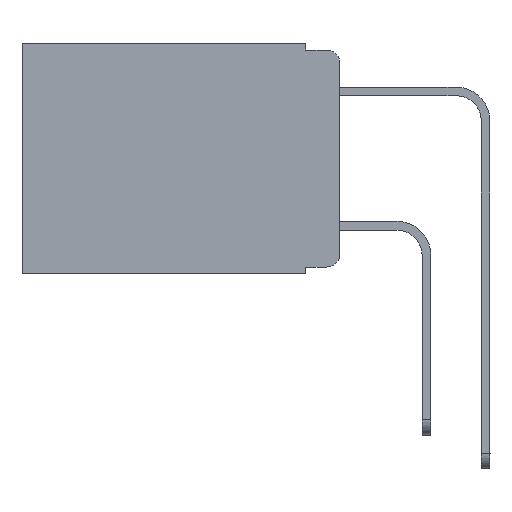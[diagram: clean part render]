
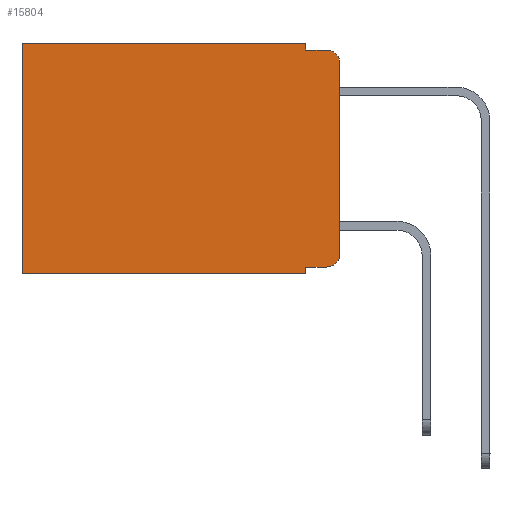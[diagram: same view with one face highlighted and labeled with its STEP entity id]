
A CAD part, left-side view. The second image highlights one B-rep face of the part: STEP entity #15804.
In plain terms, the highlighted planar face has unit normal (-1, 0, 0).
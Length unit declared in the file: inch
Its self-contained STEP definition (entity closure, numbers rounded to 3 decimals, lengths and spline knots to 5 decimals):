
#84 = PLANE ( 'NONE',  #8182 ) ;
#148 = EDGE_CURVE ( 'NONE', #10541, #10847, #10152, .T. ) ;
#207 = LINE ( 'NONE', #398, #5199 ) ;
#265 = DIRECTION ( 'NONE',  ( 0., 0., -1. ) ) ;
#279 = EDGE_CURVE ( 'NONE', #10847, #17438, #1580, .T. ) ;
#398 = CARTESIAN_POINT ( 'NONE',  ( 0.298, 0.051, -0.01 ) ) ;
#643 = LINE ( 'NONE', #9648, #5048 ) ;
#1150 = VECTOR ( 'NONE', #265, 39.37008 ) ;
#1245 = CIRCLE ( 'NONE', #7846, 0.02 ) ;
#1301 = CARTESIAN_POINT ( 'NONE',  ( 0.298, 0.02, -0.333 ) ) ;
#1580 = CIRCLE ( 'NONE', #14166, 0.02 ) ;
#1648 = VERTEX_POINT ( 'NONE', #5000 ) ;
#1787 = VERTEX_POINT ( 'NONE', #8437 ) ;
#1946 = ORIENTED_EDGE ( 'NONE', *, *, #148, .T. ) ;
#2930 = CARTESIAN_POINT ( 'NONE',  ( 0.298, 0.051, -0.333 ) ) ;
#3008 = CARTESIAN_POINT ( 'NONE',  ( 0.298, 0., 0. ) ) ;
#3046 = VECTOR ( 'NONE', #5633, 39.37008 ) ;
#3281 = CARTESIAN_POINT ( 'NONE',  ( 0.298, 0.473, 0. ) ) ;
#3369 = DIRECTION ( 'NONE',  ( 0., 1., 0. ) ) ;
#3670 = DIRECTION ( 'NONE',  ( 0., -1., 0. ) ) ;
#3976 = VERTEX_POINT ( 'NONE', #5634 ) ;
#4318 = CARTESIAN_POINT ( 'NONE',  ( 0.298, 0.051, 0. ) ) ;
#5000 = CARTESIAN_POINT ( 'NONE',  ( 0.298, 0.051, -0.01 ) ) ;
#5048 = VECTOR ( 'NONE', #16836, 39.37008 ) ;
#5199 = VECTOR ( 'NONE', #3670, 39.37008 ) ;
#5296 = LINE ( 'NONE', #8389, #6853 ) ;
#5306 = EDGE_LOOP ( 'NONE', ( #9159, #17242, #14947, #7207, #8049, #16032, #10344, #6523, #1946, #17351 ) ) ;
#5423 = VERTEX_POINT ( 'NONE', #17029 ) ;
#5633 = DIRECTION ( 'NONE',  ( 0., 1., 0. ) ) ;
#5634 = CARTESIAN_POINT ( 'NONE',  ( 0.298, 0., -0.03 ) ) ;
#5685 = DIRECTION ( 'NONE',  ( 0., 0., -1. ) ) ;
#5725 = DIRECTION ( 'NONE',  ( 0., 0., -1. ) ) ;
#6523 = ORIENTED_EDGE ( 'NONE', *, *, #9237, .F. ) ;
#6524 = CARTESIAN_POINT ( 'NONE',  ( 0.298, 0.051, -0.343 ) ) ;
#6615 = LINE ( 'NONE', #12767, #3046 ) ;
#6853 = VECTOR ( 'NONE', #18492, 39.37008 ) ;
#7080 = CARTESIAN_POINT ( 'NONE',  ( 0.298, 0.02, -0.03 ) ) ;
#7207 = ORIENTED_EDGE ( 'NONE', *, *, #15802, .F. ) ;
#7315 = DIRECTION ( 'NONE',  ( 0., 0., -1. ) ) ;
#7410 = CARTESIAN_POINT ( 'NONE',  ( 0.298, 0.02, -0.313 ) ) ;
#7846 = AXIS2_PLACEMENT_3D ( 'NONE', #7080, #12811, #5685 ) ;
#8049 = ORIENTED_EDGE ( 'NONE', *, *, #14150, .T. ) ;
#8182 = AXIS2_PLACEMENT_3D ( 'NONE', #3008, #11652, #5725 ) ;
#8389 = CARTESIAN_POINT ( 'NONE',  ( 0.298, 0., 0. ) ) ;
#8437 = CARTESIAN_POINT ( 'NONE',  ( 0.298, 0.02, -0.01 ) ) ;
#8621 = FACE_OUTER_BOUND ( 'NONE', #5306, .T. ) ;
#8739 = DIRECTION ( 'NONE',  ( 0., -1., 0. ) ) ;
#8832 = DIRECTION ( 'NONE',  ( -1., 0., 0. ) ) ;
#8921 = DIRECTION ( 'NONE',  ( 0., 0., -1. ) ) ;
#9159 = ORIENTED_EDGE ( 'NONE', *, *, #10274, .F. ) ;
#9237 = EDGE_CURVE ( 'NONE', #10541, #10205, #643, .T. ) ;
#9374 = VERTEX_POINT ( 'NONE', #12197 ) ;
#9648 = CARTESIAN_POINT ( 'NONE',  ( 0.298, 0.051, 0. ) ) ;
#9680 = CARTESIAN_POINT ( 'NONE',  ( 0.298, 0., -0.313 ) ) ;
#10079 = CARTESIAN_POINT ( 'NONE',  ( 0.298, 0.473, -0.343 ) ) ;
#10152 = LINE ( 'NONE', #2930, #15358 ) ;
#10205 = VERTEX_POINT ( 'NONE', #6524 ) ;
#10274 = EDGE_CURVE ( 'NONE', #3976, #17438, #5296, .T. ) ;
#10344 = ORIENTED_EDGE ( 'NONE', *, *, #14481, .F. ) ;
#10541 = VERTEX_POINT ( 'NONE', #16104 ) ;
#10570 = VERTEX_POINT ( 'NONE', #10079 ) ;
#10847 = VERTEX_POINT ( 'NONE', #1301 ) ;
#11604 = EDGE_CURVE ( 'NONE', #9374, #10570, #17503, .T. ) ;
#11652 = DIRECTION ( 'NONE',  ( 1., 0., 0. ) ) ;
#12197 = CARTESIAN_POINT ( 'NONE',  ( 0.298, 0.473, 0. ) ) ;
#12767 = CARTESIAN_POINT ( 'NONE',  ( 0.298, 0., 0. ) ) ;
#12811 = DIRECTION ( 'NONE',  ( -1., 0., 0. ) ) ;
#12927 = VECTOR ( 'NONE', #3369, 39.37008 ) ;
#14150 = EDGE_CURVE ( 'NONE', #5423, #9374, #6615, .T. ) ;
#14166 = AXIS2_PLACEMENT_3D ( 'NONE', #7410, #8832, #8921 ) ;
#14481 = EDGE_CURVE ( 'NONE', #10205, #10570, #16261, .T. ) ;
#14947 = ORIENTED_EDGE ( 'NONE', *, *, #16036, .F. ) ;
#15027 = CARTESIAN_POINT ( 'NONE',  ( 0.298, 0., -0.343 ) ) ;
#15181 = EDGE_CURVE ( 'NONE', #3976, #1787, #1245, .T. ) ;
#15358 = VECTOR ( 'NONE', #8739, 39.37008 ) ;
#15802 = EDGE_CURVE ( 'NONE', #5423, #1648, #17313, .T. ) ;
#15804 = ADVANCED_FACE ( 'NONE', ( #8621 ), #84, .F. ) ;
#16032 = ORIENTED_EDGE ( 'NONE', *, *, #11604, .T. ) ;
#16036 = EDGE_CURVE ( 'NONE', #1648, #1787, #207, .T. ) ;
#16104 = CARTESIAN_POINT ( 'NONE',  ( 0.298, 0.051, -0.333 ) ) ;
#16261 = LINE ( 'NONE', #15027, #12927 ) ;
#16306 = VECTOR ( 'NONE', #7315, 39.37008 ) ;
#16836 = DIRECTION ( 'NONE',  ( 0., 0., -1. ) ) ;
#17029 = CARTESIAN_POINT ( 'NONE',  ( 0.298, 0.051, 0. ) ) ;
#17242 = ORIENTED_EDGE ( 'NONE', *, *, #15181, .T. ) ;
#17313 = LINE ( 'NONE', #4318, #16306 ) ;
#17351 = ORIENTED_EDGE ( 'NONE', *, *, #279, .T. ) ;
#17438 = VERTEX_POINT ( 'NONE', #9680 ) ;
#17503 = LINE ( 'NONE', #3281, #1150 ) ;
#18492 = DIRECTION ( 'NONE',  ( 0., 0., -1. ) ) ;
